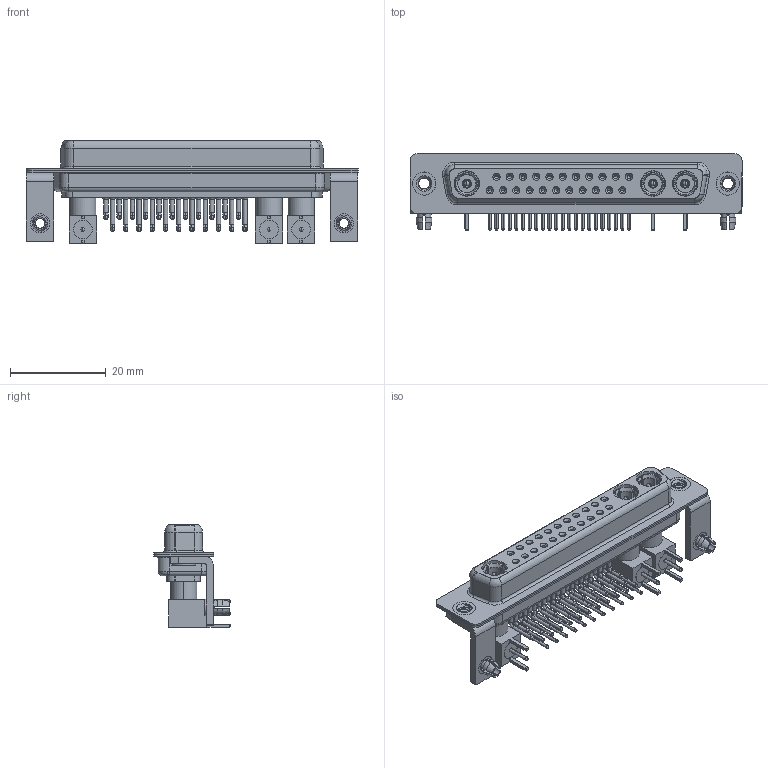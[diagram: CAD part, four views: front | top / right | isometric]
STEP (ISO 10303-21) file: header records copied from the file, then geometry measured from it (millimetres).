
FILE_DESCRIPTION (( 'STEP AP203' ), '1' );
FILE_NAME ('630-25W3640-7N3.STEP', '2022-06-07T08:34:42', ( '' ), ( '' ), 'SwSTEP 2.0', 'SolidWorks 2020', '' );
FILE_SCHEMA (( 'CONFIG_CONTROL_DESIGN' ));
Length unit declared in the file: millimetre
Products named in the file (18): Co-Ax Plug Assy_RA; Insulator Pin_Straight PC Tail; RA Back Shell; 630Combo Contact Row 1; Pin_RA; Insulator RA Pin; 630Combo Board Lock; 630-25W3640-7N3; 630Combo Shell Front_37 Contacts; 630Combo Housing_25W3; 630Combo Shell Rear_37 Contacts; Locking Collar; 630Combo Stabilizer Bracket; 630Combo Contact Row 2; Co-Ax Plug_RA PC Tail; 630Combo Threaded Rivet_3
Assembly tree (52 placements, depth 3):
  630-25W3640-7N3
    630Combo Housing_25W3
    630Combo Shell Front_37 Contacts
    630Combo Shell Rear_37 Contacts
    630Combo Threaded Rivet_3  x2
    630Combo Stabilizer Bracket  x2
    630Combo Board Lock  x2
    Co-Ax Plug Assy_RA
      Co-Ax Plug_RA PC Tail
      Insulator Pin_Straight PC Tail
      Pin_RA
      Locking Collar
      RA Back Shell
      Insulator RA Pin
    Co-Ax Plug Assy_RA
      Co-Ax Plug_RA PC Tail
      Insulator Pin_Straight PC Tail
      Pin_RA
      Locking Collar
      RA Back Shell
      Insulator RA Pin
    Co-Ax Plug Assy_RA
      Co-Ax Plug_RA PC Tail
      Insulator Pin_Straight PC Tail
      Pin_RA
      Locking Collar
      RA Back Shell
      Insulator RA Pin
    630Combo Contact Row 1  x11
    630Combo Contact Row 2  x11
Bounding box: 69.4 x 16 x 21.41 mm (x, y, z)
Volume: 6476.8 mm3; surface area: 15377.2 mm2
Topology: 49 solids, 49 shells, 2081 faces, 5208 edges, 3280 vertices
Faces by surface type: cylinder 888, plane 666, cone 343, bspline 97, torus 75, sphere 12
Entity records: 29795 total; most frequent: CARTESIAN_POINT 6260, DIRECTION 4748, ORIENTED_EDGE 4028, EDGE_CURVE 2014, AXIS2_PLACEMENT_3D 1953, VERTEX_POINT 1285, CIRCLE 1051, EDGE_LOOP 1033
